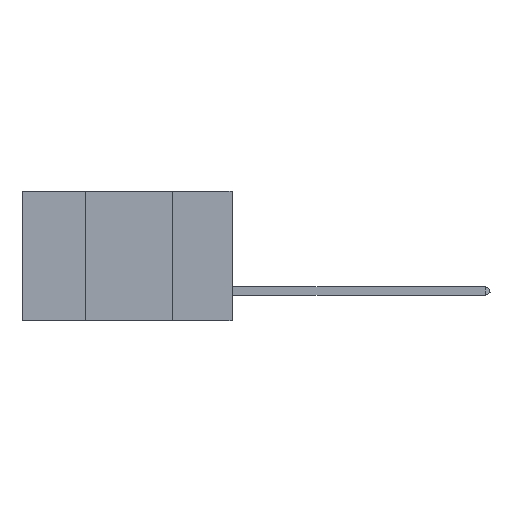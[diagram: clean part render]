
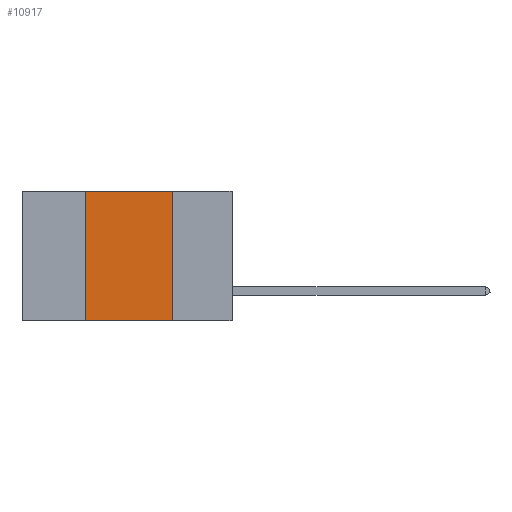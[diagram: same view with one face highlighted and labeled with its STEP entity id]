
A CAD part, left-side view. The second image highlights one B-rep face of the part: STEP entity #10917.
In plain terms, the highlighted planar face has unit normal (-1, 0, 0).
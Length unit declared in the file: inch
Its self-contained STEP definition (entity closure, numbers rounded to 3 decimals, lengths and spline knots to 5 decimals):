
#337 = CARTESIAN_POINT ( 'NONE',  ( 0., 0.42, 0. ) ) ;
#1709 = EDGE_CURVE ( 'NONE', #4134, #20779, #19900, .T. ) ;
#3076 = DIRECTION ( 'NONE',  ( 0., 0., -1. ) ) ;
#3222 = VECTOR ( 'NONE', #21436, 39.37008 ) ;
#3534 = DIRECTION ( 'NONE',  ( 0., 0., -1. ) ) ;
#3678 = VERTEX_POINT ( 'NONE', #13291 ) ;
#4134 = VERTEX_POINT ( 'NONE', #23542 ) ;
#4877 = EDGE_LOOP ( 'NONE', ( #18436, #12760, #6504, #14856 ) ) ;
#5661 = CARTESIAN_POINT ( 'NONE',  ( 0., 0.6, -0.37 ) ) ;
#6504 = ORIENTED_EDGE ( 'NONE', *, *, #6703, .F. ) ;
#6703 = EDGE_CURVE ( 'NONE', #3678, #4134, #9648, .T. ) ;
#6832 = CARTESIAN_POINT ( 'NONE',  ( 0., 0.17, 0. ) ) ;
#8358 = VECTOR ( 'NONE', #3076, 39.37008 ) ;
#8657 = LINE ( 'NONE', #10718, #8358 ) ;
#9317 = DIRECTION ( 'NONE',  ( 0., -1., 0. ) ) ;
#9648 = LINE ( 'NONE', #337, #9973 ) ;
#9973 = VECTOR ( 'NONE', #20140, 39.37008 ) ;
#10718 = CARTESIAN_POINT ( 'NONE',  ( 0., 0.17, 0. ) ) ;
#10877 = VECTOR ( 'NONE', #9317, 39.37008 ) ;
#10917 = ADVANCED_FACE ( 'NONE', ( #19920 ), #15416, .F. ) ;
#12760 = ORIENTED_EDGE ( 'NONE', *, *, #1709, .F. ) ;
#12770 = EDGE_CURVE ( 'NONE', #3678, #24101, #14908, .T. ) ;
#13291 = CARTESIAN_POINT ( 'NONE',  ( 0., 0.42, -0.37 ) ) ;
#14856 = ORIENTED_EDGE ( 'NONE', *, *, #12770, .T. ) ;
#14908 = LINE ( 'NONE', #5661, #10877 ) ;
#15416 = PLANE ( 'NONE',  #23014 ) ;
#18436 = ORIENTED_EDGE ( 'NONE', *, *, #21281, .F. ) ;
#19900 = LINE ( 'NONE', #21268, #3222 ) ;
#19920 = FACE_OUTER_BOUND ( 'NONE', #4877, .T. ) ;
#20140 = DIRECTION ( 'NONE',  ( 0., 0., 1. ) ) ;
#20779 = VERTEX_POINT ( 'NONE', #6832 ) ;
#21268 = CARTESIAN_POINT ( 'NONE',  ( 0., 0.6, 0. ) ) ;
#21281 = EDGE_CURVE ( 'NONE', #20779, #24101, #8657, .T. ) ;
#21436 = DIRECTION ( 'NONE',  ( 0., -1., 0. ) ) ;
#23014 = AXIS2_PLACEMENT_3D ( 'NONE', #23331, #25411, #3534 ) ;
#23331 = CARTESIAN_POINT ( 'NONE',  ( 0., 0.6, 0. ) ) ;
#23482 = CARTESIAN_POINT ( 'NONE',  ( 0., 0.17, -0.37 ) ) ;
#23542 = CARTESIAN_POINT ( 'NONE',  ( 0., 0.42, 0. ) ) ;
#24101 = VERTEX_POINT ( 'NONE', #23482 ) ;
#25411 = DIRECTION ( 'NONE',  ( 1., 0., 0. ) ) ;
